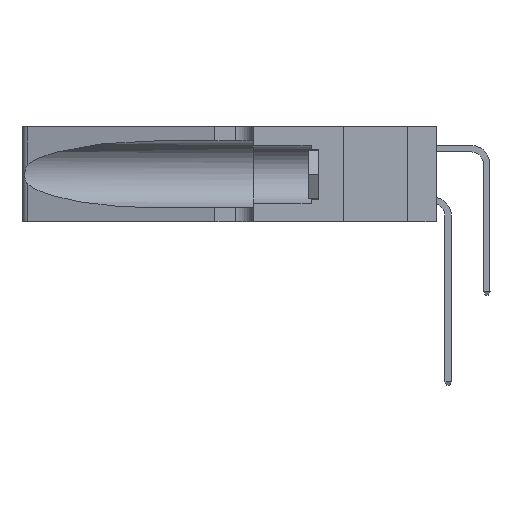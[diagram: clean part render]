
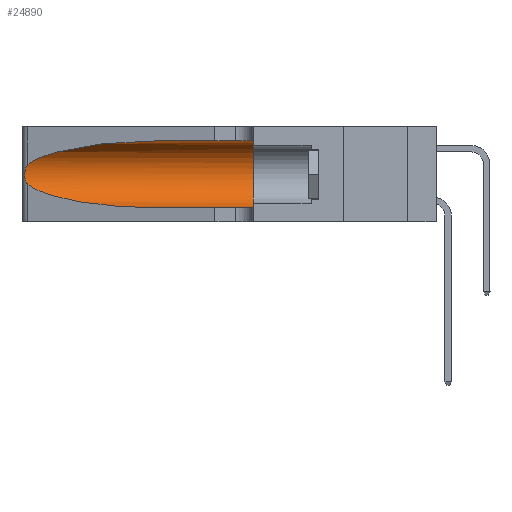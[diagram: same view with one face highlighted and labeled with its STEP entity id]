
A CAD part, left-side view. The second image highlights one B-rep face of the part: STEP entity #24890.
In plain terms, the highlighted cylindrical face has radius 3.308 mm (diameter 6.617 mm), a partial arc.
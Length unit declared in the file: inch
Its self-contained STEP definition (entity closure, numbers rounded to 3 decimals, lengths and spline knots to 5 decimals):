
#312 = DIRECTION ( 'NONE',  ( 0., -1., 0. ) ) ;
#574 = VERTEX_POINT ( 'NONE', #37639 ) ;
#724 = DIRECTION ( 'NONE',  ( 0., 0., -1. ) ) ;
#1597 = CARTESIAN_POINT ( 'NONE',  ( 0.25487, 1.22718, 0.14631 ) ) ;
#3311 = CARTESIAN_POINT ( 'NONE',  ( 0.25555, 1.22994, 0.2215 ) ) ;
#3706 = CARTESIAN_POINT ( 'NONE',  ( 0.25487, 1.22718, 0.22369 ) ) ;
#3774 = VECTOR ( 'NONE', #312, 39.37008 ) ;
#3864 = EDGE_LOOP ( 'NONE', ( #9901, #3928, #37691, #14223, #24992, #33084 ) ) ;
#3928 = ORIENTED_EDGE ( 'NONE', *, *, #21927, .T. ) ;
#4217 =( BOUNDED_CURVE ( )  B_SPLINE_CURVE ( 3, ( #5686, #36600, #24236, #27651 ),
 .UNSPECIFIED., .F., .F. ) 
 B_SPLINE_CURVE_WITH_KNOTS ( ( 4, 4 ),
 ( 1.5708, 2.84003 ),
 .UNSPECIFIED. ) 
 CURVE ( )  GEOMETRIC_REPRESENTATION_ITEM ( )  RATIONAL_B_SPLINE_CURVE ( ( 1., 0.87, 0.87, 1. ) ) 
 REPRESENTATION_ITEM ( '' )  );
#4961 = CARTESIAN_POINT ( 'NONE',  ( 0.18966, 0.96281, 0.05475 ) ) ;
#5686 = CARTESIAN_POINT ( 'NONE',  ( 0.1305, 0.72297, 0.31525 ) ) ;
#5836 = CARTESIAN_POINT ( 'NONE',  ( 0.1305, 1.61858, 0.05475 ) ) ;
#5884 = DIRECTION ( 'NONE',  ( 0., 0., 1. ) ) ;
#6157 = DIRECTION ( 'NONE',  ( 0., 1., 0. ) ) ;
#6693 = CARTESIAN_POINT ( 'NONE',  ( 0.1305, 0.72297, 0.31525 ) ) ;
#6730 = CARTESIAN_POINT ( 'NONE',  ( 0.26075, 1.23896, 0.19203 ) ) ;
#7276 = CARTESIAN_POINT ( 'NONE',  ( 0.25487, 1.22718, 0.14631 ) ) ;
#7464 = CARTESIAN_POINT ( 'NONE',  ( 0.1305, 1.61858, 0.185 ) ) ;
#9901 = ORIENTED_EDGE ( 'NONE', *, *, #36667, .T. ) ;
#10174 = VERTEX_POINT ( 'NONE', #35910 ) ;
#10995 = VECTOR ( 'NONE', #30572, 39.37008 ) ;
#11596 = CYLINDRICAL_SURFACE ( 'NONE', #31686, 0.13025 ) ;
#14223 = ORIENTED_EDGE ( 'NONE', *, *, #20016, .T. ) ;
#15650 = CIRCLE ( 'NONE', #28464, 0.13025 ) ;
#16171 = CARTESIAN_POINT ( 'NONE',  ( 0.25639, 1.23186, 0.15144 ) ) ;
#16757 = CARTESIAN_POINT ( 'NONE',  ( 0.25487, 1.22718, 0.14631 ) ) ;
#19016 = LINE ( 'NONE', #19230, #3774 ) ;
#19230 = CARTESIAN_POINT ( 'NONE',  ( 0.1305, 1.61858, 0.31525 ) ) ;
#19766 = VERTEX_POINT ( 'NONE', #16757 ) ;
#20016 = EDGE_CURVE ( 'NONE', #10174, #574, #23265, .T. ) ;
#21230 = CARTESIAN_POINT ( 'NONE',  ( 0.1305, 0.35, 0.31525 ) ) ;
#21694 = EDGE_CURVE ( 'NONE', #19766, #10174, #25398, .T. ) ;
#21927 = EDGE_CURVE ( 'NONE', #32884, #19766, #23653, .T. ) ;
#22813 = CARTESIAN_POINT ( 'NONE',  ( 0.25555, 1.22993, 0.14849 ) ) ;
#23265 = LINE ( 'NONE', #5836, #10995 ) ;
#23653 = B_SPLINE_CURVE_WITH_KNOTS ( 'NONE', 3,
 ( #3706, #3311, #25987, #39214, #31207, #34880, #6730, #35014, #37553, #34492, #31451, #16171, #22813, #7276 ),
 .UNSPECIFIED., .F., .F.,
 ( 4, 2, 2, 2, 2, 2, 4 ),
 ( 0., 0.00027, 0.00053, 0.00107, 0.0016, 0.00187, 0.00214 ),
 .UNSPECIFIED. ) ;
#23793 = CARTESIAN_POINT ( 'NONE',  ( 0.2373, 1.15595, 0.08982 ) ) ;
#24236 = CARTESIAN_POINT ( 'NONE',  ( 0.2373, 1.15595, 0.28018 ) ) ;
#24890 = ADVANCED_FACE ( 'NONE', ( #37152 ), #11596, .F. ) ;
#24992 = ORIENTED_EDGE ( 'NONE', *, *, #32354, .F. ) ;
#25398 =( BOUNDED_CURVE ( )  B_SPLINE_CURVE ( 3, ( #1597, #23793, #4961, #31972 ),
 .UNSPECIFIED., .F., .F. ) 
 B_SPLINE_CURVE_WITH_KNOTS ( ( 4, 4 ),
 ( 3.44316, 4.71239 ),
 .UNSPECIFIED. ) 
 CURVE ( )  GEOMETRIC_REPRESENTATION_ITEM ( )  RATIONAL_B_SPLINE_CURVE ( ( 1., 0.87, 0.87, 1. ) ) 
 REPRESENTATION_ITEM ( '' )  );
#25987 = CARTESIAN_POINT ( 'NONE',  ( 0.25639, 1.23184, 0.21858 ) ) ;
#27447 = VERTEX_POINT ( 'NONE', #21230 ) ;
#27651 = CARTESIAN_POINT ( 'NONE',  ( 0.25487, 1.22718, 0.22369 ) ) ;
#28464 = AXIS2_PLACEMENT_3D ( 'NONE', #40660, #6157, #5884 ) ;
#30572 = DIRECTION ( 'NONE',  ( 0., -1., 0. ) ) ;
#30652 = EDGE_CURVE ( 'NONE', #35348, #27447, #19016, .T. ) ;
#31207 = CARTESIAN_POINT ( 'NONE',  ( 0.25854, 1.2359, 0.20912 ) ) ;
#31451 = CARTESIAN_POINT ( 'NONE',  ( 0.25789, 1.23486, 0.15765 ) ) ;
#31686 = AXIS2_PLACEMENT_3D ( 'NONE', #7464, #38485, #724 ) ;
#31972 = CARTESIAN_POINT ( 'NONE',  ( 0.1305, 0.72297, 0.05475 ) ) ;
#32354 = EDGE_CURVE ( 'NONE', #27447, #574, #15650, .T. ) ;
#32884 = VERTEX_POINT ( 'NONE', #33844 ) ;
#33084 = ORIENTED_EDGE ( 'NONE', *, *, #30652, .F. ) ;
#33844 = CARTESIAN_POINT ( 'NONE',  ( 0.25487, 1.22718, 0.22369 ) ) ;
#34492 = CARTESIAN_POINT ( 'NONE',  ( 0.25856, 1.23593, 0.16098 ) ) ;
#34880 = CARTESIAN_POINT ( 'NONE',  ( 0.26018, 1.23835, 0.19895 ) ) ;
#35014 = CARTESIAN_POINT ( 'NONE',  ( 0.26075, 1.23896, 0.178 ) ) ;
#35348 = VERTEX_POINT ( 'NONE', #6693 ) ;
#35910 = CARTESIAN_POINT ( 'NONE',  ( 0.1305, 0.72297, 0.05475 ) ) ;
#36600 = CARTESIAN_POINT ( 'NONE',  ( 0.18966, 0.96281, 0.31525 ) ) ;
#36667 = EDGE_CURVE ( 'NONE', #35348, #32884, #4217, .T. ) ;
#37152 = FACE_OUTER_BOUND ( 'NONE', #3864, .T. ) ;
#37553 = CARTESIAN_POINT ( 'NONE',  ( 0.26017, 1.23833, 0.17102 ) ) ;
#37639 = CARTESIAN_POINT ( 'NONE',  ( 0.1305, 0.35, 0.05475 ) ) ;
#37691 = ORIENTED_EDGE ( 'NONE', *, *, #21694, .T. ) ;
#38485 = DIRECTION ( 'NONE',  ( 0., -1., 0. ) ) ;
#39214 = CARTESIAN_POINT ( 'NONE',  ( 0.25787, 1.23484, 0.2124 ) ) ;
#40660 = CARTESIAN_POINT ( 'NONE',  ( 0.1305, 0.35, 0.185 ) ) ;
